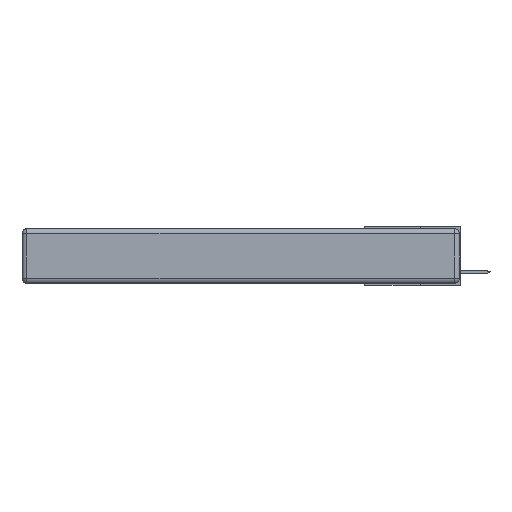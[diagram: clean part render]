
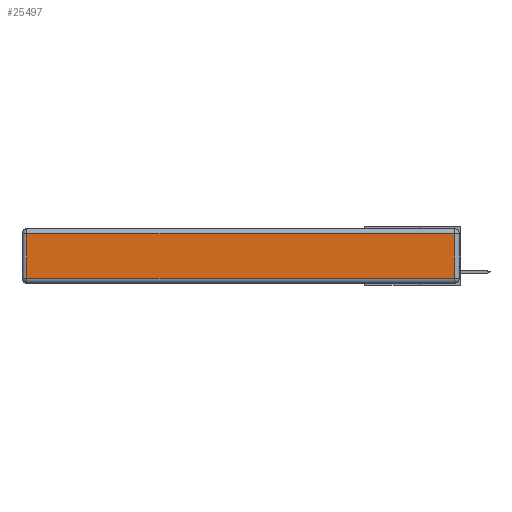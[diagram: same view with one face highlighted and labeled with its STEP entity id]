
A CAD part, left-side view. The second image highlights one B-rep face of the part: STEP entity #25497.
In plain terms, the highlighted planar face has unit normal (-1, 0, 0).
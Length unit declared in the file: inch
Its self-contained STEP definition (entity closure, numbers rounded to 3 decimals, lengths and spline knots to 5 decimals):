
#1124 = ORIENTED_EDGE ( 'NONE', *, *, #3704, .T. ) ;
#1456 = CARTESIAN_POINT ( 'NONE',  ( 0., 2.72, -0.313 ) ) ;
#1672 = DIRECTION ( 'NONE',  ( 0., 0., 1. ) ) ;
#3252 = CARTESIAN_POINT ( 'NONE',  ( 0., 2.75, -0.03 ) ) ;
#3585 = VECTOR ( 'NONE', #15699, 39.37008 ) ;
#3704 = EDGE_CURVE ( 'NONE', #21186, #27489, #11181, .T. ) ;
#3852 = DIRECTION ( 'NONE',  ( 0., 0., 1. ) ) ;
#5280 = ORIENTED_EDGE ( 'NONE', *, *, #13761, .T. ) ;
#5312 = DIRECTION ( 'NONE',  ( 0., -1., 0. ) ) ;
#8018 = CARTESIAN_POINT ( 'NONE',  ( 0., 2.72, -0.03 ) ) ;
#8595 = CARTESIAN_POINT ( 'NONE',  ( 0., 0.03, -0.343 ) ) ;
#8604 = LINE ( 'NONE', #13180, #3585 ) ;
#10187 = DIRECTION ( 'NONE',  ( 0., 1., 0. ) ) ;
#10809 = AXIS2_PLACEMENT_3D ( 'NONE', #15281, #17560, #3852 ) ;
#10984 = PLANE ( 'NONE',  #10809 ) ;
#11151 = CARTESIAN_POINT ( 'NONE',  ( 0., 0.03, -0.03 ) ) ;
#11181 = LINE ( 'NONE', #8595, #20120 ) ;
#11195 = EDGE_CURVE ( 'NONE', #11768, #21186, #22984, .T. ) ;
#11768 = VERTEX_POINT ( 'NONE', #1456 ) ;
#13180 = CARTESIAN_POINT ( 'NONE',  ( 0., 2.72, -0.343 ) ) ;
#13761 = EDGE_CURVE ( 'NONE', #27489, #25949, #27494, .T. ) ;
#15281 = CARTESIAN_POINT ( 'NONE',  ( 0., 0., -0.343 ) ) ;
#15699 = DIRECTION ( 'NONE',  ( 0., 0., -1. ) ) ;
#17553 = VECTOR ( 'NONE', #5312, 39.37008 ) ;
#17560 = DIRECTION ( 'NONE',  ( -1., 0., 0. ) ) ;
#17726 = FACE_OUTER_BOUND ( 'NONE', #18624, .T. ) ;
#18624 = EDGE_LOOP ( 'NONE', ( #25178, #1124, #5280, #29605 ) ) ;
#19838 = VECTOR ( 'NONE', #10187, 39.37008 ) ;
#20120 = VECTOR ( 'NONE', #1672, 39.37008 ) ;
#21186 = VERTEX_POINT ( 'NONE', #24927 ) ;
#22484 = EDGE_CURVE ( 'NONE', #25949, #11768, #8604, .T. ) ;
#22984 = LINE ( 'NONE', #27633, #17553 ) ;
#24927 = CARTESIAN_POINT ( 'NONE',  ( 0., 0.03, -0.313 ) ) ;
#25178 = ORIENTED_EDGE ( 'NONE', *, *, #11195, .T. ) ;
#25497 = ADVANCED_FACE ( 'NONE', ( #17726 ), #10984, .T. ) ;
#25949 = VERTEX_POINT ( 'NONE', #8018 ) ;
#27489 = VERTEX_POINT ( 'NONE', #11151 ) ;
#27494 = LINE ( 'NONE', #3252, #19838 ) ;
#27633 = CARTESIAN_POINT ( 'NONE',  ( 0., 0., -0.313 ) ) ;
#29605 = ORIENTED_EDGE ( 'NONE', *, *, #22484, .T. ) ;
